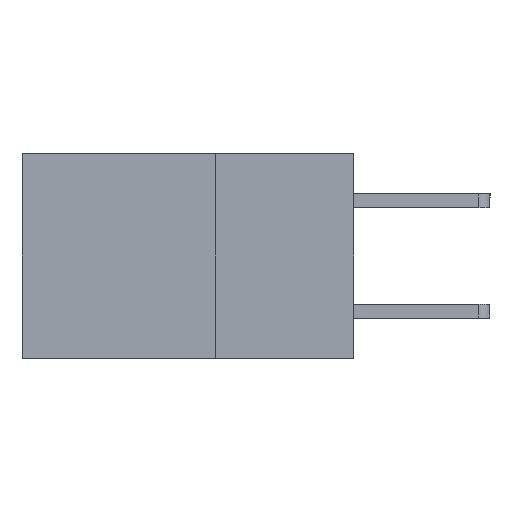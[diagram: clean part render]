
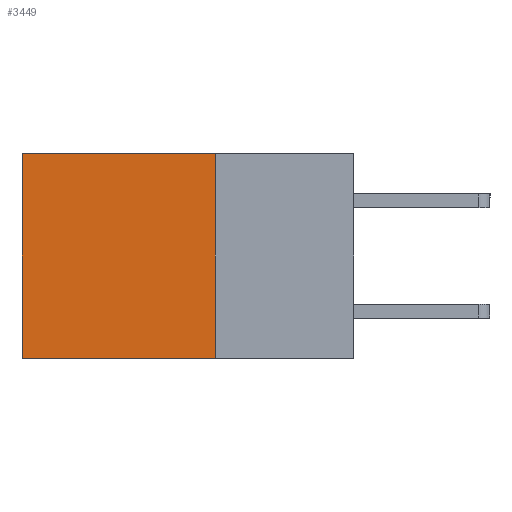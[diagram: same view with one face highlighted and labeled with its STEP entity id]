
A CAD part, left-side view. The second image highlights one B-rep face of the part: STEP entity #3449.
In plain terms, the highlighted planar face has unit normal (-1, 0, 0).
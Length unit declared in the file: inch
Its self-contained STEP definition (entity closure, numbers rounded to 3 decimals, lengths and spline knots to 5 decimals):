
#51 = DIRECTION ( 'NONE',  ( 0., 1., 0. ) ) ;
#84 = CARTESIAN_POINT ( 'NONE',  ( 0.2875, 0.25, 0. ) ) ;
#142 = CARTESIAN_POINT ( 'NONE',  ( 0.2875, 0.25, 0. ) ) ;
#223 = CARTESIAN_POINT ( 'NONE',  ( 0.2875, 0.25, -0.37 ) ) ;
#258 = DIRECTION ( 'NONE',  ( 0., 0., -1. ) ) ;
#272 = VERTEX_POINT ( 'NONE', #10172 ) ;
#363 = VERTEX_POINT ( 'NONE', #84 ) ;
#872 = EDGE_CURVE ( 'NONE', #363, #272, #1620, .T. ) ;
#877 = LINE ( 'NONE', #4971, #9916 ) ;
#1171 = DIRECTION ( 'NONE',  ( 0., 0., -1. ) ) ;
#1179 = EDGE_CURVE ( 'NONE', #363, #13033, #877, .T. ) ;
#1546 = CARTESIAN_POINT ( 'NONE',  ( 0.2875, 0.25, 0. ) ) ;
#1578 = EDGE_LOOP ( 'NONE', ( #9992, #11734, #3963, #11775 ) ) ;
#1620 = LINE ( 'NONE', #1546, #12476 ) ;
#2173 = DIRECTION ( 'NONE',  ( 1., 0., 0. ) ) ;
#3449 = ADVANCED_FACE ( 'NONE', ( #5182 ), #4192, .F. ) ;
#3505 = LINE ( 'NONE', #9740, #6730 ) ;
#3963 = ORIENTED_EDGE ( 'NONE', *, *, #872, .F. ) ;
#4192 = PLANE ( 'NONE',  #7385 ) ;
#4823 = VECTOR ( 'NONE', #12644, 39.37008 ) ;
#4971 = CARTESIAN_POINT ( 'NONE',  ( 0.2875, 0.25, 0. ) ) ;
#5182 = FACE_OUTER_BOUND ( 'NONE', #1578, .T. ) ;
#6730 = VECTOR ( 'NONE', #258, 39.37008 ) ;
#7385 = AXIS2_PLACEMENT_3D ( 'NONE', #142, #2173, #1171 ) ;
#8214 = CARTESIAN_POINT ( 'NONE',  ( 0.2875, 0.6, -0.37 ) ) ;
#9740 = CARTESIAN_POINT ( 'NONE',  ( 0.2875, 0.6, 0. ) ) ;
#9916 = VECTOR ( 'NONE', #51, 39.37008 ) ;
#9992 = ORIENTED_EDGE ( 'NONE', *, *, #12020, .T. ) ;
#10172 = CARTESIAN_POINT ( 'NONE',  ( 0.2875, 0.25, -0.37 ) ) ;
#10308 = LINE ( 'NONE', #223, #4823 ) ;
#10648 = CARTESIAN_POINT ( 'NONE',  ( 0.2875, 0.6, 0. ) ) ;
#11734 = ORIENTED_EDGE ( 'NONE', *, *, #12467, .F. ) ;
#11775 = ORIENTED_EDGE ( 'NONE', *, *, #1179, .T. ) ;
#11807 = DIRECTION ( 'NONE',  ( 0., 0., -1. ) ) ;
#12020 = EDGE_CURVE ( 'NONE', #13033, #12166, #3505, .T. ) ;
#12166 = VERTEX_POINT ( 'NONE', #8214 ) ;
#12467 = EDGE_CURVE ( 'NONE', #272, #12166, #10308, .T. ) ;
#12476 = VECTOR ( 'NONE', #11807, 39.37008 ) ;
#12644 = DIRECTION ( 'NONE',  ( 0., 1., 0. ) ) ;
#13033 = VERTEX_POINT ( 'NONE', #10648 ) ;
